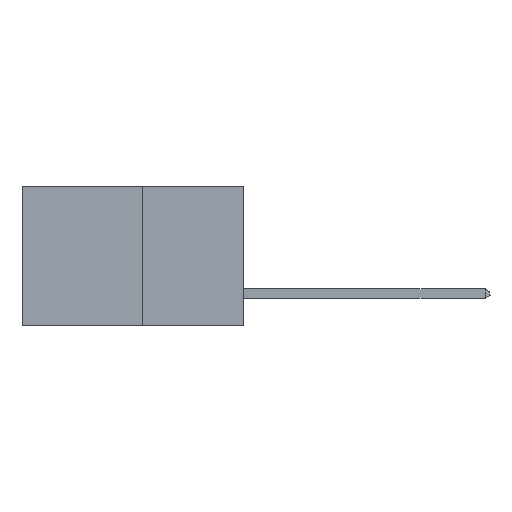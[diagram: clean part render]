
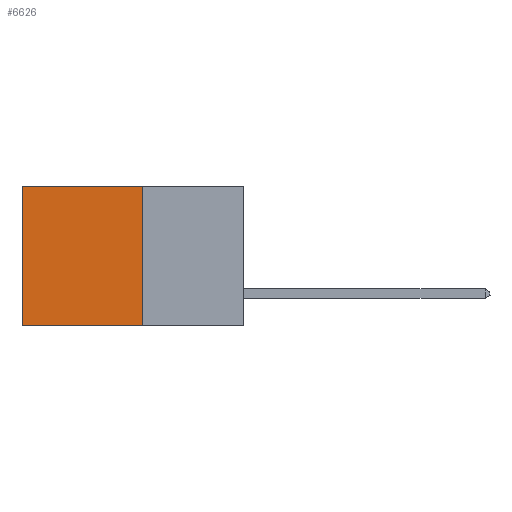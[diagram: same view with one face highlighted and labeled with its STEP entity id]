
A CAD part, left-side view. The second image highlights one B-rep face of the part: STEP entity #6626.
In plain terms, the highlighted planar face has unit normal (-1, 0, 0).
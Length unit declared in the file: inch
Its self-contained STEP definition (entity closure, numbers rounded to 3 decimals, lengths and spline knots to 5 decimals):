
#979 = CARTESIAN_POINT ( 'NONE',  ( 0.277, 0.27, -0.37 ) ) ;
#1694 = CARTESIAN_POINT ( 'NONE',  ( 0.277, 0.27, -0.37 ) ) ;
#1787 = VERTEX_POINT ( 'NONE', #979 ) ;
#2281 = VERTEX_POINT ( 'NONE', #15725 ) ;
#2732 = EDGE_CURVE ( 'NONE', #4734, #2281, #16431, .T. ) ;
#3025 = PLANE ( 'NONE',  #7985 ) ;
#3452 = DIRECTION ( 'NONE',  ( 1., 0., 0. ) ) ;
#3702 = DIRECTION ( 'NONE',  ( 0., 1., 0. ) ) ;
#3709 = CARTESIAN_POINT ( 'NONE',  ( 0.277, 0.27, -0.37 ) ) ;
#3718 = DIRECTION ( 'NONE',  ( 0., 0., -1. ) ) ;
#4090 = ORIENTED_EDGE ( 'NONE', *, *, #14760, .F. ) ;
#4517 = EDGE_LOOP ( 'NONE', ( #9916, #19388, #4090, #8150 ) ) ;
#4595 = CARTESIAN_POINT ( 'NONE',  ( 0.277, 0.59, -0.37 ) ) ;
#4734 = VERTEX_POINT ( 'NONE', #14001 ) ;
#5059 = VECTOR ( 'NONE', #3702, 39.37008 ) ;
#5112 = VECTOR ( 'NONE', #18673, 39.37008 ) ;
#5808 = CARTESIAN_POINT ( 'NONE',  ( 0.277, 0.27, 0. ) ) ;
#6626 = ADVANCED_FACE ( 'NONE', ( #17022 ), #3025, .F. ) ;
#7985 = AXIS2_PLACEMENT_3D ( 'NONE', #1694, #3452, #3718 ) ;
#8150 = ORIENTED_EDGE ( 'NONE', *, *, #14368, .T. ) ;
#8154 = LINE ( 'NONE', #3709, #5059 ) ;
#9147 = EDGE_CURVE ( 'NONE', #1787, #2281, #8154, .T. ) ;
#9613 = CARTESIAN_POINT ( 'NONE',  ( 0.277, 0.27, -0.37 ) ) ;
#9916 = ORIENTED_EDGE ( 'NONE', *, *, #2732, .T. ) ;
#10239 = DIRECTION ( 'NONE',  ( 0., 0., -1. ) ) ;
#12270 = VERTEX_POINT ( 'NONE', #17394 ) ;
#12307 = VECTOR ( 'NONE', #19419, 39.37008 ) ;
#12429 = VECTOR ( 'NONE', #10239, 39.37008 ) ;
#13218 = LINE ( 'NONE', #9613, #5112 ) ;
#14001 = CARTESIAN_POINT ( 'NONE',  ( 0.277, 0.59, 0. ) ) ;
#14368 = EDGE_CURVE ( 'NONE', #12270, #4734, #16300, .T. ) ;
#14760 = EDGE_CURVE ( 'NONE', #12270, #1787, #13218, .T. ) ;
#15725 = CARTESIAN_POINT ( 'NONE',  ( 0.277, 0.59, -0.37 ) ) ;
#16300 = LINE ( 'NONE', #5808, #12307 ) ;
#16431 = LINE ( 'NONE', #4595, #12429 ) ;
#17022 = FACE_OUTER_BOUND ( 'NONE', #4517, .T. ) ;
#17394 = CARTESIAN_POINT ( 'NONE',  ( 0.277, 0.27, 0. ) ) ;
#18673 = DIRECTION ( 'NONE',  ( 0., 0., -1. ) ) ;
#19388 = ORIENTED_EDGE ( 'NONE', *, *, #9147, .F. ) ;
#19419 = DIRECTION ( 'NONE',  ( 0., 1., 0. ) ) ;
